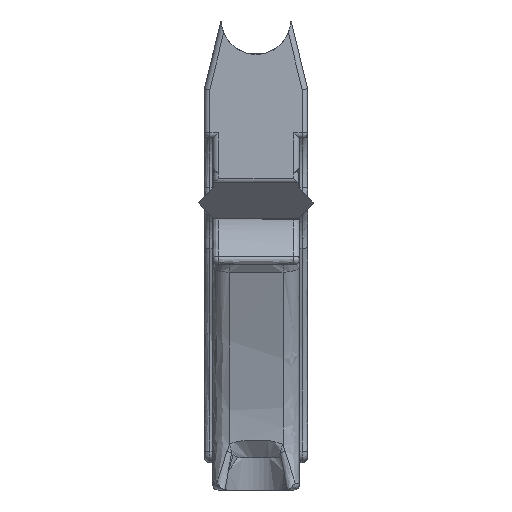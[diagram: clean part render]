
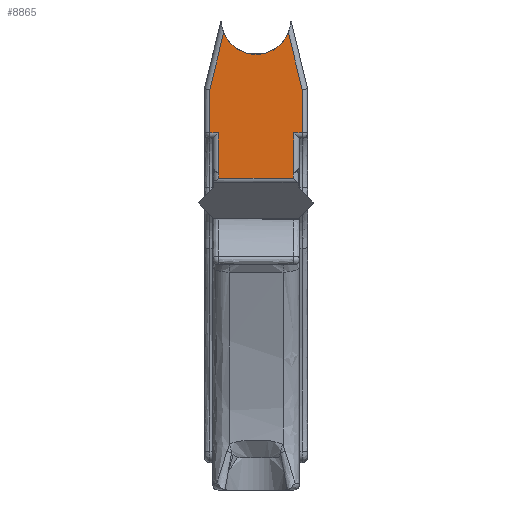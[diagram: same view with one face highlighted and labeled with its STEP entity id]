
A CAD part, front view. The second image highlights one B-rep face of the part: STEP entity #8865.
In plain terms, the highlighted planar face has unit normal (0, -1, 0).
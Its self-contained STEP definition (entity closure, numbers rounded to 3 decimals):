
#938=FACE_OUTER_BOUND('',#1431,.T.);
#1431=EDGE_LOOP('',(#7973,#7974,#7975,#7976,#7977,#7978,#7979,#7980,#7981,
#7982,#7983,#7984,#7985,#7986));
#1643=CIRCLE('',#9466,6.4);
#2439=LINE('',#18791,#3297);
#2450=LINE('',#18818,#3308);
#2460=LINE('',#18835,#3318);
#2472=LINE('',#18864,#3330);
#2473=LINE('',#18867,#3331);
#2474=LINE('',#18869,#3332);
#2475=LINE('',#18871,#3333);
#2476=LINE('',#18873,#3334);
#2477=LINE('',#18877,#3335);
#2478=LINE('',#18879,#3336);
#2479=LINE('',#18880,#3337);
#2480=LINE('',#18882,#3338);
#2481=LINE('',#18883,#3339);
#3297=VECTOR('',#11356,10.);
#3308=VECTOR('',#11383,10.);
#3318=VECTOR('',#11399,10.);
#3330=VECTOR('',#11433,10.);
#3331=VECTOR('',#11436,10.);
#3332=VECTOR('',#11437,10.);
#3333=VECTOR('',#11438,10.);
#3334=VECTOR('',#11439,10.);
#3335=VECTOR('',#11442,10.);
#3336=VECTOR('',#11443,10.);
#3337=VECTOR('',#11444,10.);
#3338=VECTOR('',#11445,1.);
#3339=VECTOR('',#11446,10.);
#4156=VERTEX_POINT('',#18787);
#4158=VERTEX_POINT('',#18790);
#4165=VERTEX_POINT('',#18815);
#4166=VERTEX_POINT('',#18817);
#4170=VERTEX_POINT('',#18834);
#4176=VERTEX_POINT('',#18862);
#4177=VERTEX_POINT('',#18866);
#4178=VERTEX_POINT('',#18868);
#4179=VERTEX_POINT('',#18870);
#4180=VERTEX_POINT('',#18872);
#4181=VERTEX_POINT('',#18874);
#4182=VERTEX_POINT('',#18876);
#4183=VERTEX_POINT('',#18878);
#4184=VERTEX_POINT('',#18881);
#5420=EDGE_CURVE('',#4158,#4156,#2439,.T.);
#5434=EDGE_CURVE('',#4166,#4165,#2450,.T.);
#5445=EDGE_CURVE('',#4166,#4170,#2460,.T.);
#5460=EDGE_CURVE('',#4176,#4165,#2472,.T.);
#5461=EDGE_CURVE('',#4177,#4156,#2473,.T.);
#5462=EDGE_CURVE('',#4178,#4177,#2474,.T.);
#5463=EDGE_CURVE('',#4179,#4178,#2475,.T.);
#5464=EDGE_CURVE('',#4180,#4179,#2476,.T.);
#5465=EDGE_CURVE('',#4180,#4181,#1643,.T.);
#5466=EDGE_CURVE('',#4182,#4181,#2477,.T.);
#5467=EDGE_CURVE('',#4183,#4182,#2478,.T.);
#5468=EDGE_CURVE('',#4170,#4183,#2479,.T.);
#5469=EDGE_CURVE('',#4184,#4176,#2480,.T.);
#5470=EDGE_CURVE('',#4158,#4184,#2481,.T.);
#7973=ORIENTED_EDGE('',*,*,#5461,.F.);
#7974=ORIENTED_EDGE('',*,*,#5462,.F.);
#7975=ORIENTED_EDGE('',*,*,#5463,.F.);
#7976=ORIENTED_EDGE('',*,*,#5464,.F.);
#7977=ORIENTED_EDGE('',*,*,#5465,.T.);
#7978=ORIENTED_EDGE('',*,*,#5466,.F.);
#7979=ORIENTED_EDGE('',*,*,#5467,.F.);
#7980=ORIENTED_EDGE('',*,*,#5468,.F.);
#7981=ORIENTED_EDGE('',*,*,#5445,.F.);
#7982=ORIENTED_EDGE('',*,*,#5434,.T.);
#7983=ORIENTED_EDGE('',*,*,#5460,.F.);
#7984=ORIENTED_EDGE('',*,*,#5469,.F.);
#7985=ORIENTED_EDGE('',*,*,#5470,.F.);
#7986=ORIENTED_EDGE('',*,*,#5420,.T.);
#8410=PLANE('',#9465);
#8865=ADVANCED_FACE('',(#938),#8410,.T.);
#9465=AXIS2_PLACEMENT_3D('',#18865,#11434,#11435);
#9466=AXIS2_PLACEMENT_3D('',#18875,#11440,#11441);
#11356=DIRECTION('',(0.707,0.,0.707));
#11383=DIRECTION('',(0.707,0.,-0.707));
#11399=DIRECTION('',(0.,0.,1.));
#11433=DIRECTION('',(0.,0.,1.));
#11434=DIRECTION('center_axis',(0.,-1.,0.));
#11435=DIRECTION('ref_axis',(1.,0.,0.));
#11436=DIRECTION('',(0.,0.,-1.));
#11437=DIRECTION('',(-1.,0.,0.));
#11438=DIRECTION('',(0.,0.,-1.));
#11439=DIRECTION('',(0.234,0.,-0.972));
#11440=DIRECTION('center_axis',(0.,1.,0.));
#11441=DIRECTION('ref_axis',(1.,0.,0.));
#11442=DIRECTION('',(0.234,0.,0.972));
#11443=DIRECTION('',(0.,0.,1.));
#11444=DIRECTION('',(-1.,0.,0.));
#11445=DIRECTION('',(-1.,0.,0.));
#11446=DIRECTION('',(0.,0.,-1.));
#18787=CARTESIAN_POINT('',(14.9,-169.,-12.));
#18790=CARTESIAN_POINT('',(14.786,-169.,-12.114));
#18791=CARTESIAN_POINT('',(15.3,-169.,-11.6));
#18815=CARTESIAN_POINT('',(1.114,-169.,-12.114));
#18817=CARTESIAN_POINT('',(1.,-169.,-12.));
#18818=CARTESIAN_POINT('',(-3.375,-169.,-7.625));
#18834=CARTESIAN_POINT('',(1.,-169.,-4.6));
#18835=CARTESIAN_POINT('',(1.,-169.,-8.575));
#18862=CARTESIAN_POINT('',(1.114,-169.,-12.908));
#18864=CARTESIAN_POINT('',(1.114,-169.,-6.143));
#18865=CARTESIAN_POINT('Origin',(15.9,-169.,2.25));
#18866=CARTESIAN_POINT('',(14.9,-169.,-4.6));
#18867=CARTESIAN_POINT('',(14.9,-169.,4.475));
#18868=CARTESIAN_POINT('',(16.4,-169.,-4.6));
#18869=CARTESIAN_POINT('',(8.675,-169.,-4.6));
#18870=CARTESIAN_POINT('',(16.4,-169.,3.381));
#18871=CARTESIAN_POINT('',(16.4,-169.,-0.213));
#18872=CARTESIAN_POINT('',(13.888,-169.,13.812));
#18873=CARTESIAN_POINT('',(15.054,-169.,8.971));
#18874=CARTESIAN_POINT('',(2.012,-169.,13.812));
#18875=CARTESIAN_POINT('Origin',(7.95,-169.,16.2));
#18876=CARTESIAN_POINT('',(-0.5,-169.,3.381));
#18877=CARTESIAN_POINT('',(-0.193,-169.,4.655));
#18878=CARTESIAN_POINT('',(-0.5,-169.,-4.6));
#18879=CARTESIAN_POINT('',(-0.5,-169.,-0.213));
#18880=CARTESIAN_POINT('',(8.675,-169.,-4.6));
#18881=CARTESIAN_POINT('',(14.786,-169.,-12.908));
#18882=CARTESIAN_POINT('',(15.786,-169.,-12.908));
#18883=CARTESIAN_POINT('',(14.786,-169.,-4.375));
